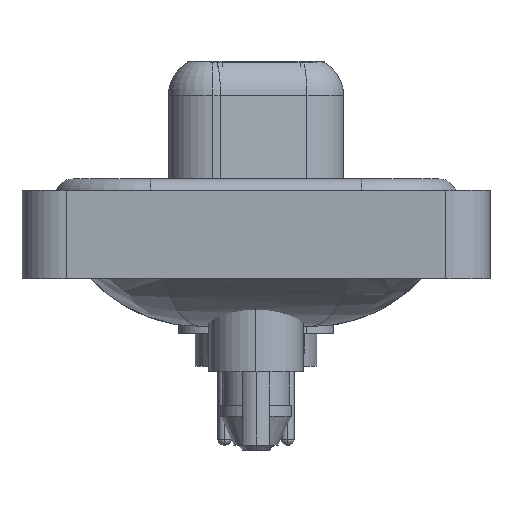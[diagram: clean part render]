
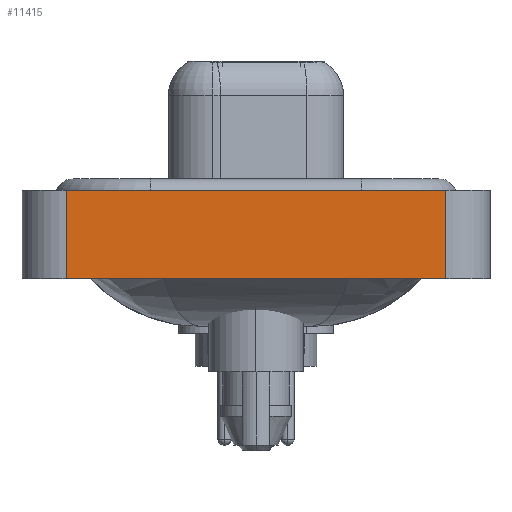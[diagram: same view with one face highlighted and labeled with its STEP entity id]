
A CAD part, left-side view. The second image highlights one B-rep face of the part: STEP entity #11415.
In plain terms, the highlighted planar face has unit normal (-1, 0, 0).
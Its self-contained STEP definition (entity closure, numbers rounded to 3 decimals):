
#714 = CARTESIAN_POINT ( 'NONE',  ( -7.35, 8.55, -3.6 ) ) ;
#780 = VERTEX_POINT ( 'NONE', #27028 ) ;
#1176 = FACE_OUTER_BOUND ( 'NONE', #9807, .T. ) ;
#1630 = CARTESIAN_POINT ( 'NONE',  ( -7.35, 8.55, 0.4 ) ) ;
#2260 = LINE ( 'NONE', #714, #3385 ) ;
#2678 = DIRECTION ( 'NONE',  ( 0., 0., 1. ) ) ;
#3385 = VECTOR ( 'NONE', #2678, 1000. ) ;
#3718 = VERTEX_POINT ( 'NONE', #22413 ) ;
#4395 = DIRECTION ( 'NONE',  ( 0., -1., 0. ) ) ;
#4463 = LINE ( 'NONE', #21596, #6581 ) ;
#4501 = ORIENTED_EDGE ( 'NONE', *, *, #14819, .T. ) ;
#5526 = PLANE ( 'NONE',  #10252 ) ;
#6397 = CARTESIAN_POINT ( 'NONE',  ( -7.35, -8.55, -3.6 ) ) ;
#6581 = VECTOR ( 'NONE', #15259, 1000. ) ;
#7907 = CARTESIAN_POINT ( 'NONE',  ( -7.35, -8.55, -3.6 ) ) ;
#7975 = EDGE_CURVE ( 'NONE', #3718, #20524, #25663, .T. ) ;
#9737 = DIRECTION ( 'NONE',  ( 0., 0., 1. ) ) ;
#9807 = EDGE_LOOP ( 'NONE', ( #12245, #25883, #23030, #4501 ) ) ;
#10252 = AXIS2_PLACEMENT_3D ( 'NONE', #7907, #27044, #9737 ) ;
#11415 = ADVANCED_FACE ( 'NONE', ( #1176 ), #5526, .T. ) ;
#12245 = ORIENTED_EDGE ( 'NONE', *, *, #7975, .T. ) ;
#12666 = LINE ( 'NONE', #23648, #15251 ) ;
#14819 = EDGE_CURVE ( 'NONE', #780, #3718, #4463, .T. ) ;
#15251 = VECTOR ( 'NONE', #4395, 1000. ) ;
#15259 = DIRECTION ( 'NONE',  ( 0., -1., 0. ) ) ;
#16501 = VERTEX_POINT ( 'NONE', #1630 ) ;
#18576 = CARTESIAN_POINT ( 'NONE',  ( -7.35, -8.55, 0.4 ) ) ;
#20524 = VERTEX_POINT ( 'NONE', #18576 ) ;
#20797 = EDGE_CURVE ( 'NONE', #780, #16501, #2260, .T. ) ;
#20881 = DIRECTION ( 'NONE',  ( 0., 0., 1. ) ) ;
#21596 = CARTESIAN_POINT ( 'NONE',  ( -7.35, -8.55, -3.6 ) ) ;
#22413 = CARTESIAN_POINT ( 'NONE',  ( -7.35, -8.55, -3.6 ) ) ;
#23030 = ORIENTED_EDGE ( 'NONE', *, *, #20797, .F. ) ;
#23648 = CARTESIAN_POINT ( 'NONE',  ( -7.35, -8.55, 0.4 ) ) ;
#25663 = LINE ( 'NONE', #6397, #25899 ) ;
#25883 = ORIENTED_EDGE ( 'NONE', *, *, #26002, .F. ) ;
#25899 = VECTOR ( 'NONE', #20881, 1000. ) ;
#26002 = EDGE_CURVE ( 'NONE', #16501, #20524, #12666, .T. ) ;
#27028 = CARTESIAN_POINT ( 'NONE',  ( -7.35, 8.55, -3.6 ) ) ;
#27044 = DIRECTION ( 'NONE',  ( -1., 0., 0. ) ) ;
